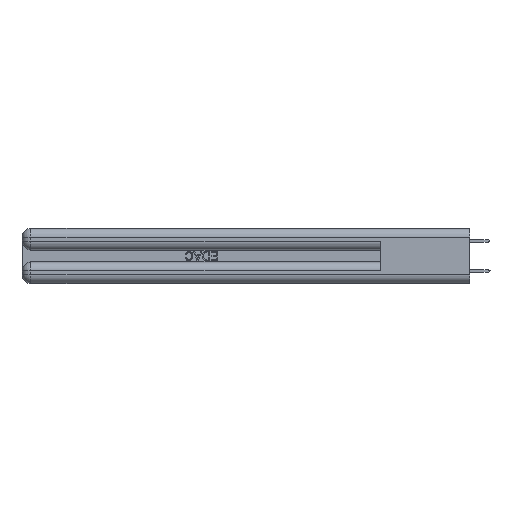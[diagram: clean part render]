
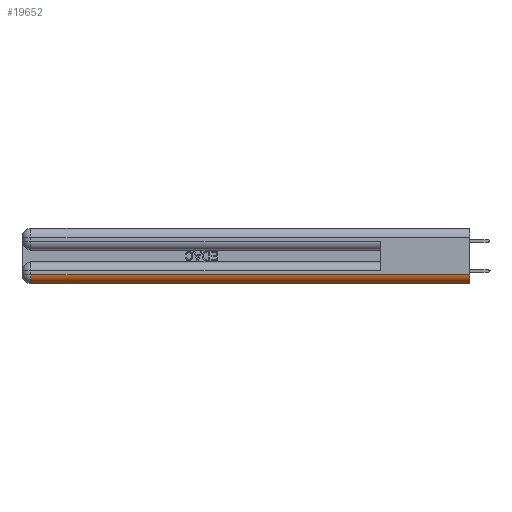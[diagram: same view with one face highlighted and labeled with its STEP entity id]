
A CAD part, left-side view. The second image highlights one B-rep face of the part: STEP entity #19652.
In plain terms, the highlighted cylindrical face has radius 1.524 mm (diameter 3.048 mm), a partial arc.
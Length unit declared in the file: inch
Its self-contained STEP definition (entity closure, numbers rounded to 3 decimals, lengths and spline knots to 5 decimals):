
#22 = CIRCLE ( 'NONE', #29274, 0.06 ) ;
#2587 = ORIENTED_EDGE ( 'NONE', *, *, #12105, .F. ) ;
#3686 = VERTEX_POINT ( 'NONE', #19882 ) ;
#4305 = CARTESIAN_POINT ( 'NONE',  ( 0.06, 0., 0.06 ) ) ;
#5791 = EDGE_CURVE ( 'NONE', #3686, #20320, #22, .T. ) ;
#6291 = VECTOR ( 'NONE', #25837, 39.37008 ) ;
#6562 = DIRECTION ( 'NONE',  ( 0., 1., 0. ) ) ;
#6697 = ORIENTED_EDGE ( 'NONE', *, *, #36274, .F. ) ;
#6703 = DIRECTION ( 'NONE',  ( 0., 1., 0. ) ) ;
#8180 = CARTESIAN_POINT ( 'NONE',  ( 0., 2.94, 0.06 ) ) ;
#9836 = DIRECTION ( 'NONE',  ( 0., 0., 1. ) ) ;
#10245 = CIRCLE ( 'NONE', #35220, 0.06 ) ;
#10354 = CARTESIAN_POINT ( 'NONE',  ( 0.06, 3., 0. ) ) ;
#12105 = EDGE_CURVE ( 'NONE', #17597, #3686, #17476, .T. ) ;
#13773 = VECTOR ( 'NONE', #6562, 39.37008 ) ;
#15680 = CARTESIAN_POINT ( 'NONE',  ( 0., 0., 0.06 ) ) ;
#17476 = LINE ( 'NONE', #10354, #13773 ) ;
#17597 = VERTEX_POINT ( 'NONE', #42945 ) ;
#17724 = EDGE_CURVE ( 'NONE', #36713, #17597, #10245, .T. ) ;
#19652 = ADVANCED_FACE ( 'NONE', ( #33738 ), #26616, .T. ) ;
#19882 = CARTESIAN_POINT ( 'NONE',  ( 0.06, 2.94, 0. ) ) ;
#20320 = VERTEX_POINT ( 'NONE', #8180 ) ;
#21802 = DIRECTION ( 'NONE',  ( 0., -1., 0. ) ) ;
#25837 = DIRECTION ( 'NONE',  ( 0., -1., 0. ) ) ;
#26616 = CYLINDRICAL_SURFACE ( 'NONE', #36698, 0.06 ) ;
#27569 = CARTESIAN_POINT ( 'NONE',  ( 0.06, 2.94, 0.06 ) ) ;
#27804 = DIRECTION ( 'NONE',  ( 0., 0., 1. ) ) ;
#29274 = AXIS2_PLACEMENT_3D ( 'NONE', #27569, #41840, #27804 ) ;
#33395 = CARTESIAN_POINT ( 'NONE',  ( 0., 0., 0.06 ) ) ;
#33738 = FACE_OUTER_BOUND ( 'NONE', #34294, .T. ) ;
#34294 = EDGE_LOOP ( 'NONE', ( #36171, #6697, #39682, #2587 ) ) ;
#35220 = AXIS2_PLACEMENT_3D ( 'NONE', #4305, #21802, #35435 ) ;
#35435 = DIRECTION ( 'NONE',  ( 0., 0., 1. ) ) ;
#36081 = LINE ( 'NONE', #33395, #6291 ) ;
#36171 = ORIENTED_EDGE ( 'NONE', *, *, #17724, .F. ) ;
#36274 = EDGE_CURVE ( 'NONE', #20320, #36713, #36081, .T. ) ;
#36655 = CARTESIAN_POINT ( 'NONE',  ( 0.06, 0., 0.06 ) ) ;
#36698 = AXIS2_PLACEMENT_3D ( 'NONE', #36655, #6703, #9836 ) ;
#36713 = VERTEX_POINT ( 'NONE', #15680 ) ;
#39682 = ORIENTED_EDGE ( 'NONE', *, *, #5791, .F. ) ;
#41840 = DIRECTION ( 'NONE',  ( 0., 1., 0. ) ) ;
#42945 = CARTESIAN_POINT ( 'NONE',  ( 0.06, 0., 0. ) ) ;
